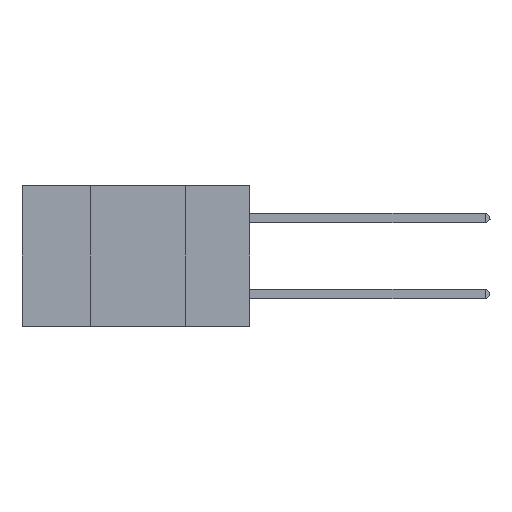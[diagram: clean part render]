
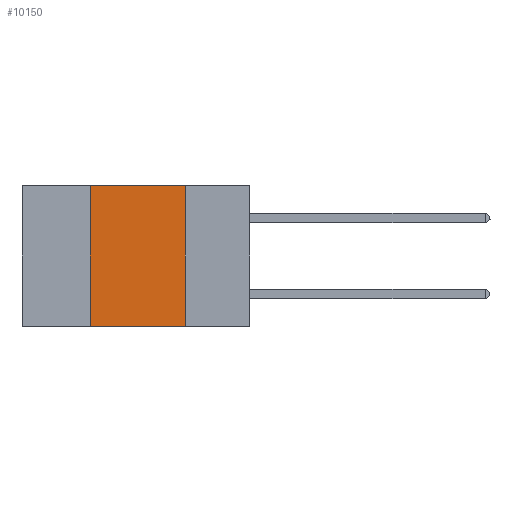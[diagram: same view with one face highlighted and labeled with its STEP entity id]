
A CAD part, left-side view. The second image highlights one B-rep face of the part: STEP entity #10150.
In plain terms, the highlighted planar face has unit normal (-1, 0, 0).
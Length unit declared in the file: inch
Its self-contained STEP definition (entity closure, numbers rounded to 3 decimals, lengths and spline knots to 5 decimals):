
#5 = DIRECTION ( 'NONE',  ( 0., -1., 0. ) ) ;
#712 = VERTEX_POINT ( 'NONE', #14305 ) ;
#887 = DIRECTION ( 'NONE',  ( 0., -1., 0. ) ) ;
#2301 = LINE ( 'NONE', #6921, #17042 ) ;
#2531 = CARTESIAN_POINT ( 'NONE',  ( 0., 0.42, 0. ) ) ;
#3040 = LINE ( 'NONE', #11973, #11165 ) ;
#3562 = ORIENTED_EDGE ( 'NONE', *, *, #11102, .F. ) ;
#3730 = CARTESIAN_POINT ( 'NONE',  ( 0., 0.17, 0. ) ) ;
#4695 = DIRECTION ( 'NONE',  ( 0., 0., 1. ) ) ;
#5091 = CARTESIAN_POINT ( 'NONE',  ( 0., 0.42, 0. ) ) ;
#5145 = LINE ( 'NONE', #3730, #12505 ) ;
#5803 = CARTESIAN_POINT ( 'NONE',  ( 0., 0.42, -0.37 ) ) ;
#6695 = AXIS2_PLACEMENT_3D ( 'NONE', #19816, #11944, #16685 ) ;
#6921 = CARTESIAN_POINT ( 'NONE',  ( 0., 0.6, 0. ) ) ;
#7244 = EDGE_LOOP ( 'NONE', ( #3562, #18974, #9482, #10234 ) ) ;
#7330 = FACE_OUTER_BOUND ( 'NONE', #7244, .T. ) ;
#7947 = DIRECTION ( 'NONE',  ( 0., 0., -1. ) ) ;
#9396 = LINE ( 'NONE', #5091, #18929 ) ;
#9482 = ORIENTED_EDGE ( 'NONE', *, *, #10737, .F. ) ;
#9595 = VERTEX_POINT ( 'NONE', #2531 ) ;
#9603 = EDGE_CURVE ( 'NONE', #17574, #16562, #3040, .T. ) ;
#10150 = ADVANCED_FACE ( 'NONE', ( #7330 ), #10334, .F. ) ;
#10234 = ORIENTED_EDGE ( 'NONE', *, *, #9603, .T. ) ;
#10334 = PLANE ( 'NONE',  #6695 ) ;
#10737 = EDGE_CURVE ( 'NONE', #17574, #9595, #9396, .T. ) ;
#11102 = EDGE_CURVE ( 'NONE', #712, #16562, #5145, .T. ) ;
#11165 = VECTOR ( 'NONE', #5, 39.37008 ) ;
#11944 = DIRECTION ( 'NONE',  ( 1., 0., 0. ) ) ;
#11973 = CARTESIAN_POINT ( 'NONE',  ( 0., 0.6, -0.37 ) ) ;
#12505 = VECTOR ( 'NONE', #7947, 39.37008 ) ;
#14156 = EDGE_CURVE ( 'NONE', #9595, #712, #2301, .T. ) ;
#14305 = CARTESIAN_POINT ( 'NONE',  ( 0., 0.17, 0. ) ) ;
#16535 = CARTESIAN_POINT ( 'NONE',  ( 0., 0.17, -0.37 ) ) ;
#16562 = VERTEX_POINT ( 'NONE', #16535 ) ;
#16685 = DIRECTION ( 'NONE',  ( 0., 0., -1. ) ) ;
#17042 = VECTOR ( 'NONE', #887, 39.37008 ) ;
#17574 = VERTEX_POINT ( 'NONE', #5803 ) ;
#18929 = VECTOR ( 'NONE', #4695, 39.37008 ) ;
#18974 = ORIENTED_EDGE ( 'NONE', *, *, #14156, .F. ) ;
#19816 = CARTESIAN_POINT ( 'NONE',  ( 0., 0.6, 0. ) ) ;
